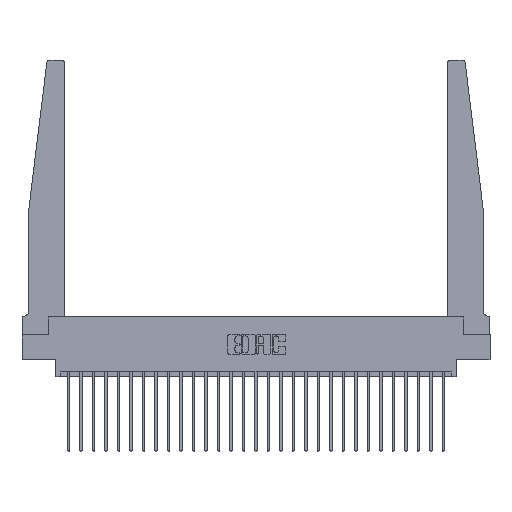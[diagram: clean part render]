
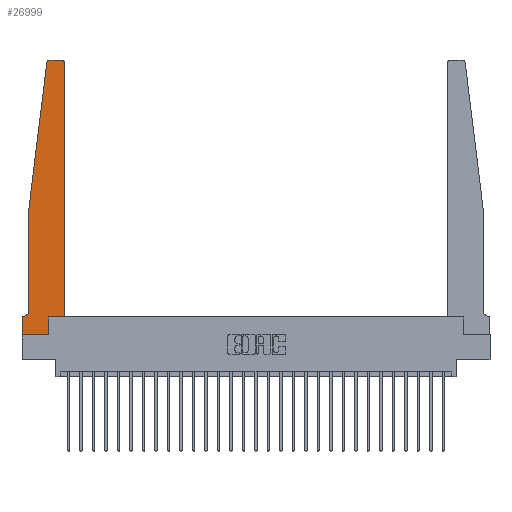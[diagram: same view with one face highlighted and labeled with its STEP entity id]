
A CAD part, top view. The second image highlights one B-rep face of the part: STEP entity #26999.
In plain terms, the highlighted planar face has unit normal (0, 0, 1).
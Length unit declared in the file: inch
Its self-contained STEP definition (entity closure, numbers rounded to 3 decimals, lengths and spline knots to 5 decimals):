
#293 = LINE ( 'NONE', #6746, #16318 ) ;
#695 = CARTESIAN_POINT ( 'NONE',  ( 0.2605, 0.18, 0.37 ) ) ;
#1139 = CARTESIAN_POINT ( 'NONE',  ( 0.425, 0.18, 0.37 ) ) ;
#1704 = CARTESIAN_POINT ( 'NONE',  ( 0.065, 1.25, 0.37 ) ) ;
#1818 = DIRECTION ( 'NONE',  ( 0., 1., 0. ) ) ;
#2207 = CARTESIAN_POINT ( 'NONE',  ( 0.015, 0.2375, 0.37 ) ) ;
#2312 = VECTOR ( 'NONE', #10107, 39.37008 ) ;
#2324 = VECTOR ( 'NONE', #1818, 39.37008 ) ;
#2752 = EDGE_CURVE ( 'NONE', #21926, #22835, #293, .T. ) ;
#2920 = CIRCLE ( 'NONE', #16482, 0.03 ) ;
#3112 = EDGE_CURVE ( 'NONE', #12300, #13165, #18567, .T. ) ;
#3178 = ORIENTED_EDGE ( 'NONE', *, *, #17524, .T. ) ;
#3251 = CARTESIAN_POINT ( 'NONE',  ( 0.065, 1.25, 0.37 ) ) ;
#3258 = CIRCLE ( 'NONE', #3687, 0.05 ) ;
#3428 = ORIENTED_EDGE ( 'NONE', *, *, #7700, .T. ) ;
#3646 = VECTOR ( 'NONE', #7052, 39.37008 ) ;
#3687 = AXIS2_PLACEMENT_3D ( 'NONE', #2207, #4257, #23463 ) ;
#3919 = DIRECTION ( 'NONE',  ( 0., 0., 1. ) ) ;
#4049 = CARTESIAN_POINT ( 'NONE',  ( 0., 0.1875, 0.37 ) ) ;
#4090 = CARTESIAN_POINT ( 'NONE',  ( 0.2605, 0., 0.37 ) ) ;
#4182 = DIRECTION ( 'NONE',  ( 0., 0., 1. ) ) ;
#4257 = DIRECTION ( 'NONE',  ( 0., 0., -1. ) ) ;
#4429 = DIRECTION ( 'NONE',  ( 0., -1., 0. ) ) ;
#4988 = EDGE_CURVE ( 'NONE', #26792, #13446, #3258, .T. ) ;
#5253 = VECTOR ( 'NONE', #22924, 39.37008 ) ;
#5976 = CARTESIAN_POINT ( 'NONE',  ( 0.065, 0.2375, 0.37 ) ) ;
#6130 = EDGE_CURVE ( 'NONE', #16802, #12300, #11959, .T. ) ;
#6197 = CARTESIAN_POINT ( 'NONE',  ( 0.27653, 2.75, 0.37 ) ) ;
#6202 = CARTESIAN_POINT ( 'NONE',  ( 0.425, 0.18, 0.37 ) ) ;
#6529 = DIRECTION ( 'NONE',  ( 1., 0., 0. ) ) ;
#6746 = CARTESIAN_POINT ( 'NONE',  ( 0., 0., 0.37 ) ) ;
#6900 = CARTESIAN_POINT ( 'NONE',  ( 0., 0., 0.37 ) ) ;
#7052 = DIRECTION ( 'NONE',  ( -1., 0., 0. ) ) ;
#7285 = LINE ( 'NONE', #695, #17254 ) ;
#7672 = AXIS2_PLACEMENT_3D ( 'NONE', #18385, #20044, #26721 ) ;
#7700 = EDGE_CURVE ( 'NONE', #13446, #19361, #21582, .T. ) ;
#7795 = DIRECTION ( 'NONE',  ( -1., 0., 0. ) ) ;
#8274 = EDGE_CURVE ( 'NONE', #22835, #16802, #7285, .T. ) ;
#8362 = ORIENTED_EDGE ( 'NONE', *, *, #8714, .T. ) ;
#8714 = EDGE_CURVE ( 'NONE', #17156, #18380, #15884, .T. ) ;
#9622 = ORIENTED_EDGE ( 'NONE', *, *, #3112, .T. ) ;
#9631 = CARTESIAN_POINT ( 'NONE',  ( 0.24675, 2.72367, 0.37 ) ) ;
#9789 = EDGE_CURVE ( 'NONE', #18380, #18207, #19927, .T. ) ;
#10107 = DIRECTION ( 'NONE',  ( -0.122, -0.992, 0. ) ) ;
#10418 = EDGE_CURVE ( 'NONE', #18207, #16170, #16418, .T. ) ;
#10635 = CARTESIAN_POINT ( 'NONE',  ( 0., 0., 0.37 ) ) ;
#11894 = EDGE_CURVE ( 'NONE', #16170, #26792, #20516, .T. ) ;
#11909 = CARTESIAN_POINT ( 'NONE',  ( 0.425, 2.72, 0.37 ) ) ;
#11959 = LINE ( 'NONE', #6202, #5253 ) ;
#12300 = VERTEX_POINT ( 'NONE', #1139 ) ;
#12602 = ORIENTED_EDGE ( 'NONE', *, *, #8274, .T. ) ;
#12694 = CARTESIAN_POINT ( 'NONE',  ( 0.395, 2.72, 0.37 ) ) ;
#12824 = PLANE ( 'NONE',  #26257 ) ;
#12953 = FACE_OUTER_BOUND ( 'NONE', #14901, .T. ) ;
#13165 = VERTEX_POINT ( 'NONE', #11909 ) ;
#13204 = CARTESIAN_POINT ( 'NONE',  ( 0.065, 0.1875, 0.37 ) ) ;
#13309 = DIRECTION ( 'NONE',  ( 0., 1., 0. ) ) ;
#13446 = VERTEX_POINT ( 'NONE', #21996 ) ;
#14827 = VECTOR ( 'NONE', #26254, 39.37008 ) ;
#14901 = EDGE_LOOP ( 'NONE', ( #8362, #16124, #24931, #25034, #23090, #3428, #18886, #18596, #12602, #23170, #9622, #3178 ) ) ;
#15884 = LINE ( 'NONE', #19876, #22125 ) ;
#16124 = ORIENTED_EDGE ( 'NONE', *, *, #9789, .T. ) ;
#16170 = VERTEX_POINT ( 'NONE', #3251 ) ;
#16318 = VECTOR ( 'NONE', #25504, 39.37008 ) ;
#16418 = LINE ( 'NONE', #25041, #2312 ) ;
#16482 = AXIS2_PLACEMENT_3D ( 'NONE', #12694, #3919, #25297 ) ;
#16532 = CARTESIAN_POINT ( 'NONE',  ( 0.2605, 0.18, 0.37 ) ) ;
#16802 = VERTEX_POINT ( 'NONE', #16532 ) ;
#16872 = EDGE_CURVE ( 'NONE', #19361, #21926, #25258, .T. ) ;
#17156 = VERTEX_POINT ( 'NONE', #23046 ) ;
#17254 = VECTOR ( 'NONE', #13309, 39.37008 ) ;
#17524 = EDGE_CURVE ( 'NONE', #13165, #17156, #2920, .T. ) ;
#18207 = VERTEX_POINT ( 'NONE', #9631 ) ;
#18380 = VERTEX_POINT ( 'NONE', #6197 ) ;
#18385 = CARTESIAN_POINT ( 'NONE',  ( 0.27653, 2.72, 0.37 ) ) ;
#18567 = LINE ( 'NONE', #20770, #2324 ) ;
#18596 = ORIENTED_EDGE ( 'NONE', *, *, #2752, .T. ) ;
#18886 = ORIENTED_EDGE ( 'NONE', *, *, #16872, .T. ) ;
#19361 = VERTEX_POINT ( 'NONE', #22134 ) ;
#19876 = CARTESIAN_POINT ( 'NONE',  ( 0.25, 2.75, 0.37 ) ) ;
#19927 = CIRCLE ( 'NONE', #7672, 0.03 ) ;
#20044 = DIRECTION ( 'NONE',  ( 0., 0., 1. ) ) ;
#20516 = LINE ( 'NONE', #1704, #14827 ) ;
#20770 = CARTESIAN_POINT ( 'NONE',  ( 0.425, 0.18, 0.37 ) ) ;
#21582 = LINE ( 'NONE', #13204, #3646 ) ;
#21926 = VERTEX_POINT ( 'NONE', #10635 ) ;
#21996 = CARTESIAN_POINT ( 'NONE',  ( 0.015, 0.1875, 0.37 ) ) ;
#22125 = VECTOR ( 'NONE', #7795, 39.37008 ) ;
#22134 = CARTESIAN_POINT ( 'NONE',  ( 0., 0.1875, 0.37 ) ) ;
#22710 = VECTOR ( 'NONE', #4429, 39.37008 ) ;
#22835 = VERTEX_POINT ( 'NONE', #4090 ) ;
#22924 = DIRECTION ( 'NONE',  ( 1., 0., 0. ) ) ;
#23046 = CARTESIAN_POINT ( 'NONE',  ( 0.395, 2.75, 0.37 ) ) ;
#23090 = ORIENTED_EDGE ( 'NONE', *, *, #4988, .T. ) ;
#23170 = ORIENTED_EDGE ( 'NONE', *, *, #6130, .T. ) ;
#23463 = DIRECTION ( 'NONE',  ( -1., 0., 0. ) ) ;
#24931 = ORIENTED_EDGE ( 'NONE', *, *, #10418, .T. ) ;
#25034 = ORIENTED_EDGE ( 'NONE', *, *, #11894, .T. ) ;
#25041 = CARTESIAN_POINT ( 'NONE',  ( 0.065, 1.25, 0.37 ) ) ;
#25258 = LINE ( 'NONE', #6900, #22710 ) ;
#25297 = DIRECTION ( 'NONE',  ( 1., 0., 0. ) ) ;
#25504 = DIRECTION ( 'NONE',  ( 1., 0., 0. ) ) ;
#26254 = DIRECTION ( 'NONE',  ( 0., -1., 0. ) ) ;
#26257 = AXIS2_PLACEMENT_3D ( 'NONE', #4049, #4182, #6529 ) ;
#26721 = DIRECTION ( 'NONE',  ( 1., 0., 0. ) ) ;
#26792 = VERTEX_POINT ( 'NONE', #5976 ) ;
#26999 = ADVANCED_FACE ( 'NONE', ( #12953 ), #12824, .T. ) ;
